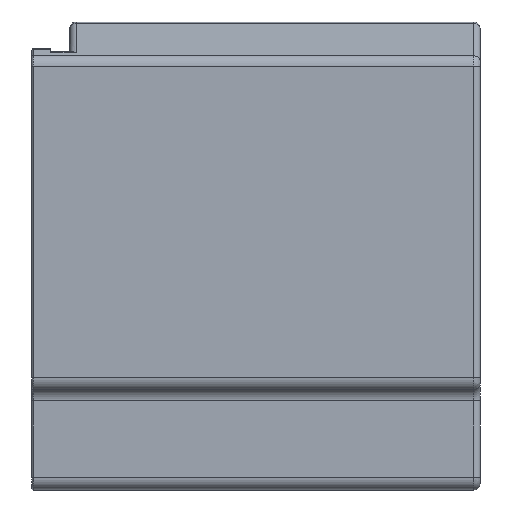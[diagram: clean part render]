
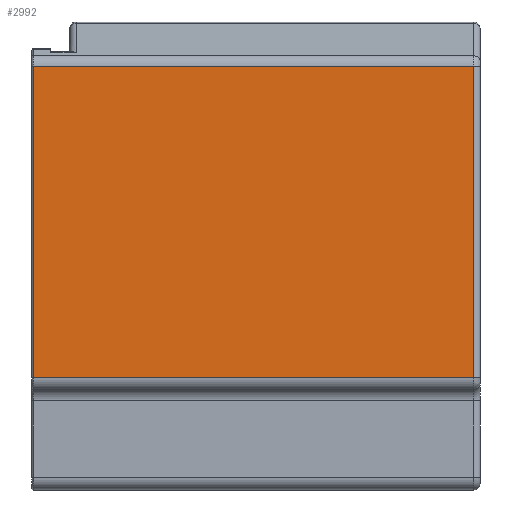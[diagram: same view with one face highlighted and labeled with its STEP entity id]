
A CAD part, left-side view. The second image highlights one B-rep face of the part: STEP entity #2992.
In plain terms, the highlighted planar face has unit normal (-1, 0, 0).
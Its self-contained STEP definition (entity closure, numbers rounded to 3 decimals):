
#43=PLANE('',#3237);
#164=FACE_OUTER_BOUND('',#361,.T.);
#361=EDGE_LOOP('',(#2050,#2051,#2052,#2053));
#552=LINE('',#4812,#781);
#562=LINE('',#4849,#791);
#563=LINE('',#4853,#792);
#564=LINE('',#4854,#793);
#781=VECTOR('',#3701,10.);
#791=VECTOR('',#3733,10.);
#792=VECTOR('',#3738,10.);
#793=VECTOR('',#3739,10.);
#1254=VERTEX_POINT('',#4804);
#1256=VERTEX_POINT('',#4810);
#1263=VERTEX_POINT('',#4848);
#1264=VERTEX_POINT('',#4852);
#1540=EDGE_CURVE('',#1256,#1254,#552,.T.);
#1555=EDGE_CURVE('',#1254,#1263,#562,.T.);
#1557=EDGE_CURVE('',#1264,#1256,#563,.T.);
#1558=EDGE_CURVE('',#1263,#1264,#564,.T.);
#2050=ORIENTED_EDGE('',*,*,#1540,.F.);
#2051=ORIENTED_EDGE('',*,*,#1557,.F.);
#2052=ORIENTED_EDGE('',*,*,#1558,.F.);
#2053=ORIENTED_EDGE('',*,*,#1555,.F.);
#2992=ADVANCED_FACE('',(#164),#43,.T.);
#3237=AXIS2_PLACEMENT_3D('',#4851,#3736,#3737);
#3701=DIRECTION('',(0.,0.,-1.));
#3733=DIRECTION('',(0.,1.,0.));
#3736=DIRECTION('center_axis',(-1.,0.,0.));
#3737=DIRECTION('ref_axis',(0.,0.,1.));
#3738=DIRECTION('',(0.,-1.,0.));
#3739=DIRECTION('',(0.,0.,1.));
#4804=CARTESIAN_POINT('',(-15.675,31.,-18.95));
#4810=CARTESIAN_POINT('',(-15.675,31.,30.347));
#4812=CARTESIAN_POINT('',(-15.675,31.,-11.288));
#4848=CARTESIAN_POINT('',(-15.675,100.75,-18.95));
#4849=CARTESIAN_POINT('',(-15.675,0.,-18.95));
#4851=CARTESIAN_POINT('Origin',(-15.675,0.,-20.95));
#4852=CARTESIAN_POINT('',(-15.675,100.75,30.347));
#4853=CARTESIAN_POINT('',(-15.675,0.,30.347));
#4854=CARTESIAN_POINT('',(-15.675,100.75,-11.288));
